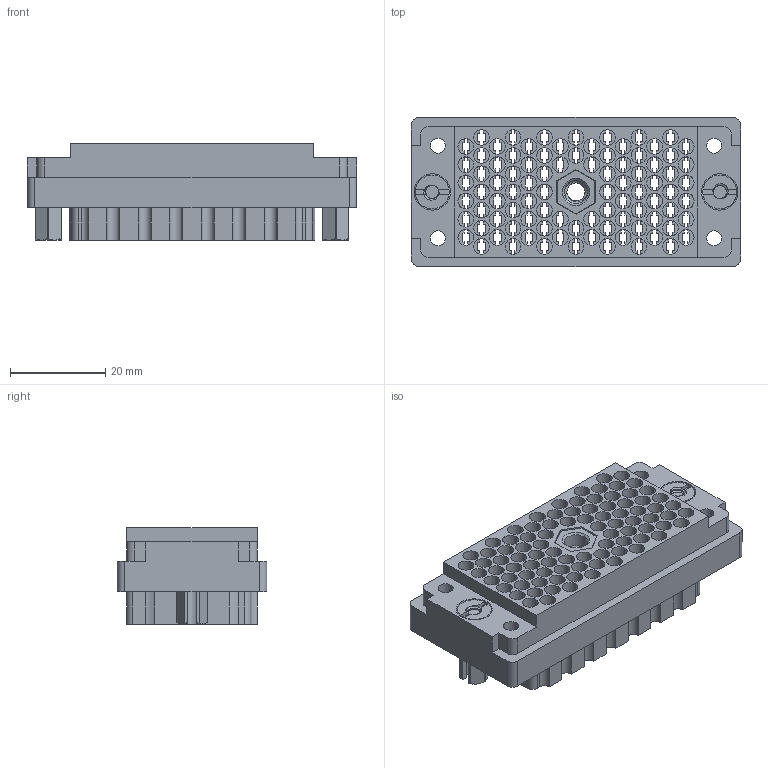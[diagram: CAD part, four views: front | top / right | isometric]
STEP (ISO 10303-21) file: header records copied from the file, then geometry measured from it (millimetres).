
FILE_DESCRIPTION (( 'STEP AP203' ), '1' );
FILE_NAME ('516-090-000-602.STEP', '2020-03-06T16:47:15', ( '' ), ( '' ), 'SwSTEP 2.0', 'SolidWorks 2016', '' );
FILE_SCHEMA (( 'CONFIG_CONTROL_DESIGN' ));
Length unit declared in the file: inch
Products named in the file (6): 516-090-000-602; 516-252-095-100; 516-221-090-102_091; 516-221-090-102_090; 516-252-091-102; 516 Part Receptacle_090
Assembly tree (6 placements, depth 2):
  516-090-000-602
    516 Part Receptacle_090
    516-252-091-102  x2
    516-221-090-102_090
    516-252-095-100
    516-221-090-102_091
Bounding box: 69.04 x 31.34 x 20.27 mm (x, y, z)
Volume: 20550 mm3; surface area: 31089.6 mm2
Topology: 6 solids, 6 shells, 2131 faces, 6267 edges, 4165 vertices
Faces by surface type: plane 1432, cylinder 625, cone 46, bspline 28
Entity records: 78110 total; most frequent: CARTESIAN_POINT 19992, ORIENTED_EDGE 12370, DIRECTION 11746, EDGE_CURVE 6185, VECTOR 4406, LINE 4406, VERTEX_POINT 4113, AXIS2_PLACEMENT_3D 3670
